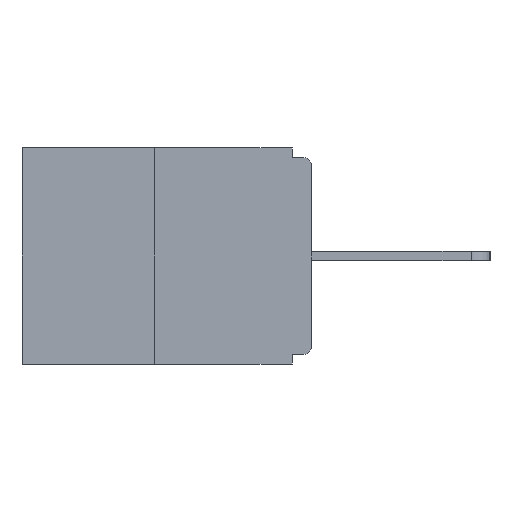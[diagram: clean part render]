
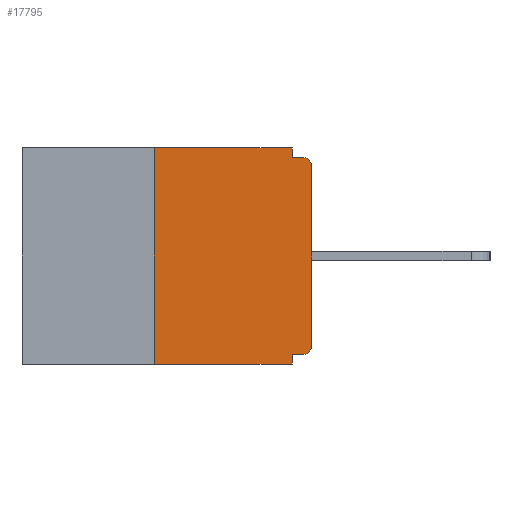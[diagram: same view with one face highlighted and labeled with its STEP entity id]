
A CAD part, left-side view. The second image highlights one B-rep face of the part: STEP entity #17795.
In plain terms, the highlighted planar face has unit normal (-1, 0, 0).
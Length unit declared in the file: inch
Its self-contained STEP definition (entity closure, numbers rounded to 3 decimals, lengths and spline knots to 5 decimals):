
#779 = DIRECTION ( 'NONE',  ( -1., 0., 0. ) ) ;
#892 = CARTESIAN_POINT ( 'NONE',  ( 0., 0.031, 0. ) ) ;
#1315 = ORIENTED_EDGE ( 'NONE', *, *, #10456, .T. ) ;
#1964 = EDGE_CURVE ( 'NONE', #6800, #8194, #11042, .T. ) ;
#2332 = CARTESIAN_POINT ( 'NONE',  ( 0., 0.015, -0.328 ) ) ;
#2421 = VERTEX_POINT ( 'NONE', #10489 ) ;
#3707 = ORIENTED_EDGE ( 'NONE', *, *, #12644, .F. ) ;
#3788 = AXIS2_PLACEMENT_3D ( 'NONE', #4384, #19064, #6585 ) ;
#3859 = CARTESIAN_POINT ( 'NONE',  ( 0., 0., -0.015 ) ) ;
#4322 = CIRCLE ( 'NONE', #9354, 0.015 ) ;
#4384 = CARTESIAN_POINT ( 'NONE',  ( 0., 0.46, 0. ) ) ;
#5642 = EDGE_CURVE ( 'NONE', #16849, #8194, #7113, .T. ) ;
#6380 = DIRECTION ( 'NONE',  ( 0., 0., -1. ) ) ;
#6585 = DIRECTION ( 'NONE',  ( 0., 0., -1. ) ) ;
#6697 = EDGE_CURVE ( 'NONE', #15985, #6881, #4322, .T. ) ;
#6800 = VERTEX_POINT ( 'NONE', #18532 ) ;
#6881 = VERTEX_POINT ( 'NONE', #13034 ) ;
#7113 = LINE ( 'NONE', #18331, #22889 ) ;
#8194 = VERTEX_POINT ( 'NONE', #24624 ) ;
#8313 = EDGE_CURVE ( 'NONE', #6800, #2421, #24578, .T. ) ;
#8432 = ORIENTED_EDGE ( 'NONE', *, *, #6697, .T. ) ;
#8546 = VERTEX_POINT ( 'NONE', #18194 ) ;
#9084 = ORIENTED_EDGE ( 'NONE', *, *, #15146, .F. ) ;
#9354 = AXIS2_PLACEMENT_3D ( 'NONE', #15258, #15235, #18365 ) ;
#9393 = VERTEX_POINT ( 'NONE', #2332 ) ;
#9531 = EDGE_CURVE ( 'NONE', #9393, #8546, #26707, .T. ) ;
#9909 = VECTOR ( 'NONE', #19032, 39.37008 ) ;
#10456 = EDGE_CURVE ( 'NONE', #8546, #15985, #16093, .T. ) ;
#10489 = CARTESIAN_POINT ( 'NONE',  ( 0., 0.25, 0. ) ) ;
#10555 = VECTOR ( 'NONE', #12141, 39.37008 ) ;
#10785 = ORIENTED_EDGE ( 'NONE', *, *, #5642, .F. ) ;
#11042 = LINE ( 'NONE', #26510, #21269 ) ;
#11431 = ORIENTED_EDGE ( 'NONE', *, *, #25878, .F. ) ;
#11866 = FACE_OUTER_BOUND ( 'NONE', #18406, .T. ) ;
#11944 = CARTESIAN_POINT ( 'NONE',  ( 0., 0.46, 0. ) ) ;
#12141 = DIRECTION ( 'NONE',  ( 0., 0., 1. ) ) ;
#12644 = EDGE_CURVE ( 'NONE', #2421, #26293, #14639, .T. ) ;
#13034 = CARTESIAN_POINT ( 'NONE',  ( 0., 0.015, -0.015 ) ) ;
#13632 = CARTESIAN_POINT ( 'NONE',  ( 0., 0.015, -0.313 ) ) ;
#14639 = LINE ( 'NONE', #11944, #20077 ) ;
#14951 = PLANE ( 'NONE',  #3788 ) ;
#14986 = ORIENTED_EDGE ( 'NONE', *, *, #8313, .F. ) ;
#15015 = CARTESIAN_POINT ( 'NONE',  ( 0., 0., -0.328 ) ) ;
#15146 = EDGE_CURVE ( 'NONE', #18546, #6881, #17738, .T. ) ;
#15235 = DIRECTION ( 'NONE',  ( -1., 0., 0. ) ) ;
#15258 = CARTESIAN_POINT ( 'NONE',  ( 0., 0.015, -0.03 ) ) ;
#15452 = LINE ( 'NONE', #15015, #9909 ) ;
#15708 = DIRECTION ( 'NONE',  ( 0., 0., -1. ) ) ;
#15985 = VERTEX_POINT ( 'NONE', #18883 ) ;
#16093 = LINE ( 'NONE', #16242, #10555 ) ;
#16242 = CARTESIAN_POINT ( 'NONE',  ( 0., 0., 0. ) ) ;
#16546 = DIRECTION ( 'NONE',  ( 0., -1., 0. ) ) ;
#16849 = VERTEX_POINT ( 'NONE', #17622 ) ;
#16851 = CARTESIAN_POINT ( 'NONE',  ( 0., 0.031, 0. ) ) ;
#17591 = ORIENTED_EDGE ( 'NONE', *, *, #9531, .T. ) ;
#17622 = CARTESIAN_POINT ( 'NONE',  ( 0., 0.031, -0.328 ) ) ;
#17738 = LINE ( 'NONE', #3859, #23035 ) ;
#17795 = ADVANCED_FACE ( 'NONE', ( #11866 ), #14951, .F. ) ;
#18110 = EDGE_CURVE ( 'NONE', #26293, #18546, #21114, .T. ) ;
#18194 = CARTESIAN_POINT ( 'NONE',  ( 0., 0., -0.313 ) ) ;
#18331 = CARTESIAN_POINT ( 'NONE',  ( 0., 0.031, -0.343 ) ) ;
#18365 = DIRECTION ( 'NONE',  ( 0., 0., -1. ) ) ;
#18406 = EDGE_LOOP ( 'NONE', ( #3707, #14986, #21013, #10785, #11431, #17591, #1315, #8432, #9084, #20104 ) ) ;
#18532 = CARTESIAN_POINT ( 'NONE',  ( 0., 0.25, -0.343 ) ) ;
#18546 = VERTEX_POINT ( 'NONE', #18679 ) ;
#18620 = VECTOR ( 'NONE', #6380, 39.37008 ) ;
#18679 = CARTESIAN_POINT ( 'NONE',  ( 0., 0.031, -0.015 ) ) ;
#18694 = VECTOR ( 'NONE', #22996, 39.37008 ) ;
#18883 = CARTESIAN_POINT ( 'NONE',  ( 0., 0., -0.03 ) ) ;
#18939 = DIRECTION ( 'NONE',  ( 0., 0., -1. ) ) ;
#19032 = DIRECTION ( 'NONE',  ( 0., 1., 0. ) ) ;
#19064 = DIRECTION ( 'NONE',  ( 1., 0., 0. ) ) ;
#20077 = VECTOR ( 'NONE', #24075, 39.37008 ) ;
#20104 = ORIENTED_EDGE ( 'NONE', *, *, #18110, .F. ) ;
#21013 = ORIENTED_EDGE ( 'NONE', *, *, #1964, .T. ) ;
#21114 = LINE ( 'NONE', #16851, #18620 ) ;
#21269 = VECTOR ( 'NONE', #22748, 39.37008 ) ;
#22748 = DIRECTION ( 'NONE',  ( 0., -1., 0. ) ) ;
#22858 = CARTESIAN_POINT ( 'NONE',  ( 0., 0.25, 0. ) ) ;
#22889 = VECTOR ( 'NONE', #18939, 39.37008 ) ;
#22977 = AXIS2_PLACEMENT_3D ( 'NONE', #13632, #779, #15708 ) ;
#22996 = DIRECTION ( 'NONE',  ( 0., 0., 1. ) ) ;
#23035 = VECTOR ( 'NONE', #16546, 39.37008 ) ;
#24075 = DIRECTION ( 'NONE',  ( 0., -1., 0. ) ) ;
#24578 = LINE ( 'NONE', #22858, #18694 ) ;
#24624 = CARTESIAN_POINT ( 'NONE',  ( 0., 0.031, -0.343 ) ) ;
#25878 = EDGE_CURVE ( 'NONE', #9393, #16849, #15452, .T. ) ;
#26293 = VERTEX_POINT ( 'NONE', #892 ) ;
#26510 = CARTESIAN_POINT ( 'NONE',  ( 0., 0.46, -0.343 ) ) ;
#26707 = CIRCLE ( 'NONE', #22977, 0.015 ) ;
